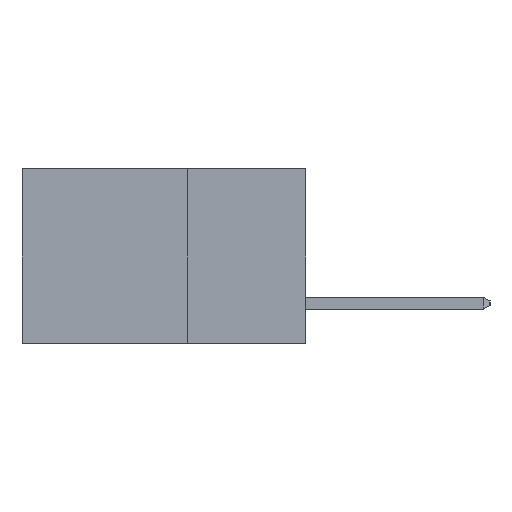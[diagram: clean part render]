
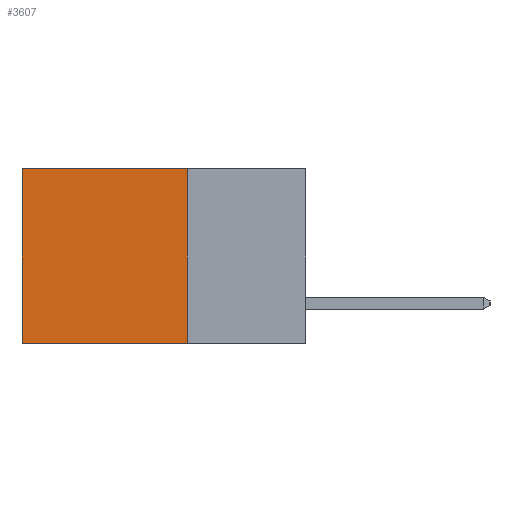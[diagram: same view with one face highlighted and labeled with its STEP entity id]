
A CAD part, left-side view. The second image highlights one B-rep face of the part: STEP entity #3607.
In plain terms, the highlighted planar face has unit normal (-1, 0, 0).
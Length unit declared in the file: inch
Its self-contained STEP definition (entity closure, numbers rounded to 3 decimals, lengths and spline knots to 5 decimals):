
#602 = VERTEX_POINT ( 'NONE', #7073 ) ;
#3205 = DIRECTION ( 'NONE',  ( 0., 1., 0. ) ) ;
#3390 = ORIENTED_EDGE ( 'NONE', *, *, #4790, .F. ) ;
#3462 = VECTOR ( 'NONE', #6508, 39.37008 ) ;
#3607 = ADVANCED_FACE ( 'NONE', ( #7415 ), #16636, .F. ) ;
#3916 = LINE ( 'NONE', #6606, #3462 ) ;
#4741 = EDGE_LOOP ( 'NONE', ( #8054, #7669, #3390, #12295 ) ) ;
#4790 = EDGE_CURVE ( 'NONE', #11499, #9068, #3916, .T. ) ;
#5237 = CARTESIAN_POINT ( 'NONE',  ( 0.2615, 0.6, 0. ) ) ;
#6382 = CARTESIAN_POINT ( 'NONE',  ( 0.2615, 0.6, -0.37 ) ) ;
#6508 = DIRECTION ( 'NONE',  ( 0., 0., -1. ) ) ;
#6606 = CARTESIAN_POINT ( 'NONE',  ( 0.2615, 0.25, -0.37 ) ) ;
#7073 = CARTESIAN_POINT ( 'NONE',  ( 0.2615, 0.6, -0.37 ) ) ;
#7415 = FACE_OUTER_BOUND ( 'NONE', #4741, .T. ) ;
#7669 = ORIENTED_EDGE ( 'NONE', *, *, #12551, .F. ) ;
#7859 = EDGE_CURVE ( 'NONE', #11499, #13988, #13769, .T. ) ;
#8007 = VECTOR ( 'NONE', #16945, 39.37008 ) ;
#8054 = ORIENTED_EDGE ( 'NONE', *, *, #12282, .T. ) ;
#9068 = VERTEX_POINT ( 'NONE', #12696 ) ;
#9803 = VECTOR ( 'NONE', #3205, 39.37008 ) ;
#10028 = CARTESIAN_POINT ( 'NONE',  ( 0.2615, 0.25, 0. ) ) ;
#10495 = VECTOR ( 'NONE', #13651, 39.37008 ) ;
#10712 = DIRECTION ( 'NONE',  ( 0., 0., -1. ) ) ;
#10788 = CARTESIAN_POINT ( 'NONE',  ( 0.2615, 0.25, -0.37 ) ) ;
#11281 = DIRECTION ( 'NONE',  ( 1., 0., 0. ) ) ;
#11488 = CARTESIAN_POINT ( 'NONE',  ( 0.2615, 0.25, 0. ) ) ;
#11499 = VERTEX_POINT ( 'NONE', #11488 ) ;
#12282 = EDGE_CURVE ( 'NONE', #13988, #602, #15465, .T. ) ;
#12295 = ORIENTED_EDGE ( 'NONE', *, *, #7859, .T. ) ;
#12339 = CARTESIAN_POINT ( 'NONE',  ( 0.2615, 0.25, -0.37 ) ) ;
#12551 = EDGE_CURVE ( 'NONE', #9068, #602, #13631, .T. ) ;
#12696 = CARTESIAN_POINT ( 'NONE',  ( 0.2615, 0.25, -0.37 ) ) ;
#13631 = LINE ( 'NONE', #12339, #10495 ) ;
#13651 = DIRECTION ( 'NONE',  ( 0., 1., 0. ) ) ;
#13769 = LINE ( 'NONE', #10028, #9803 ) ;
#13988 = VERTEX_POINT ( 'NONE', #5237 ) ;
#15449 = AXIS2_PLACEMENT_3D ( 'NONE', #10788, #11281, #10712 ) ;
#15465 = LINE ( 'NONE', #6382, #8007 ) ;
#16636 = PLANE ( 'NONE',  #15449 ) ;
#16945 = DIRECTION ( 'NONE',  ( 0., 0., -1. ) ) ;
